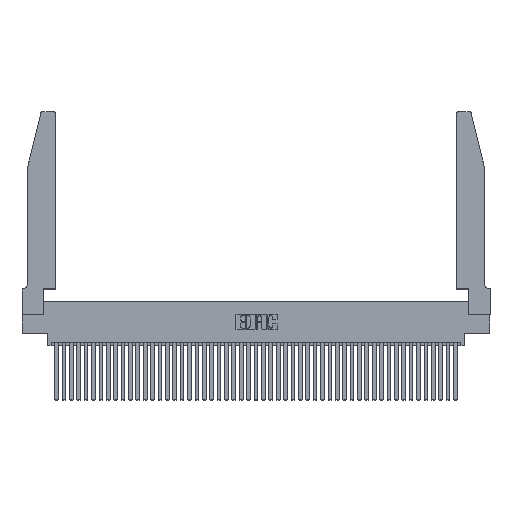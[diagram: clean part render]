
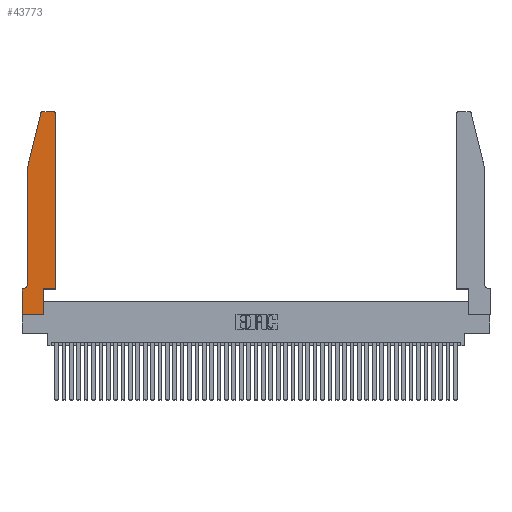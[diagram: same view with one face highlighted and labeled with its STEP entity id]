
A CAD part, top view. The second image highlights one B-rep face of the part: STEP entity #43773.
In plain terms, the highlighted planar face has unit normal (0, 0, 1).
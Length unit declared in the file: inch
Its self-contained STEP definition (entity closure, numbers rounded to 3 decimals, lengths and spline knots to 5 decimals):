
#273 = CARTESIAN_POINT ( 'NONE',  ( 0.4205, 2.75, 0.37 ) ) ;
#362 = DIRECTION ( 'NONE',  ( 0., -1., 0. ) ) ;
#999 = PLANE ( 'NONE',  #20198 ) ;
#1131 = DIRECTION ( 'NONE',  ( 0., 1., 0. ) ) ;
#1337 = DIRECTION ( 'NONE',  ( -1., 0., 0. ) ) ;
#2720 = LINE ( 'NONE', #8926, #39398 ) ;
#3730 = VECTOR ( 'NONE', #14422, 39.37008 ) ;
#4955 = DIRECTION ( 'NONE',  ( -1., 0., 0. ) ) ;
#5013 = ORIENTED_EDGE ( 'NONE', *, *, #34243, .T. ) ;
#5047 = EDGE_CURVE ( 'NONE', #11377, #32336, #18313, .T. ) ;
#5976 = VERTEX_POINT ( 'NONE', #34048 ) ;
#5987 = CARTESIAN_POINT ( 'NONE',  ( 0.2865, 0.35, 0.37 ) ) ;
#6213 = DIRECTION ( 'NONE',  ( 1., 0., 0. ) ) ;
#6577 = EDGE_CURVE ( 'NONE', #20558, #6894, #37673, .T. ) ;
#6894 = VERTEX_POINT ( 'NONE', #27374 ) ;
#7267 = VERTEX_POINT ( 'NONE', #13589 ) ;
#8099 = DIRECTION ( 'NONE',  ( -1., 0., 0. ) ) ;
#8887 = ORIENTED_EDGE ( 'NONE', *, *, #29175, .T. ) ;
#8895 = VERTEX_POINT ( 'NONE', #28972 ) ;
#8926 = CARTESIAN_POINT ( 'NONE',  ( 0.0755, 2., 0.37 ) ) ;
#9089 = ORIENTED_EDGE ( 'NONE', *, *, #15522, .T. ) ;
#9183 = LINE ( 'NONE', #5987, #32530 ) ;
#9384 = VECTOR ( 'NONE', #6213, 39.37008 ) ;
#9805 = ORIENTED_EDGE ( 'NONE', *, *, #21451, .T. ) ;
#9824 = CARTESIAN_POINT ( 'NONE',  ( 0.284, 2.72, 0.37 ) ) ;
#10603 = AXIS2_PLACEMENT_3D ( 'NONE', #9824, #34579, #20391 ) ;
#11182 = CIRCLE ( 'NONE', #27016, 0.03 ) ;
#11377 = VERTEX_POINT ( 'NONE', #30159 ) ;
#11873 = AXIS2_PLACEMENT_3D ( 'NONE', #33204, #11898, #1337 ) ;
#11898 = DIRECTION ( 'NONE',  ( 0., 0., -1. ) ) ;
#12646 = DIRECTION ( 'NONE',  ( 0., 1., 0. ) ) ;
#13589 = CARTESIAN_POINT ( 'NONE',  ( 0.2865, 0., 0.37 ) ) ;
#14422 = DIRECTION ( 'NONE',  ( -0.239, -0.971, 0. ) ) ;
#14531 = VECTOR ( 'NONE', #4955, 39.37008 ) ;
#15015 = CARTESIAN_POINT ( 'NONE',  ( 0., 0., 0.37 ) ) ;
#15304 = DIRECTION ( 'NONE',  ( 0., 0., 1. ) ) ;
#15387 = CIRCLE ( 'NONE', #11873, 0.07 ) ;
#15401 = VERTEX_POINT ( 'NONE', #40515 ) ;
#15522 = EDGE_CURVE ( 'NONE', #7267, #41668, #9183, .T. ) ;
#16374 = CIRCLE ( 'NONE', #10603, 0.03 ) ;
#17278 = ORIENTED_EDGE ( 'NONE', *, *, #20208, .T. ) ;
#18263 = DIRECTION ( 'NONE',  ( 1., 0., 0. ) ) ;
#18313 = LINE ( 'NONE', #43938, #21668 ) ;
#19512 = CARTESIAN_POINT ( 'NONE',  ( 0.4505, 0.35, 0.37 ) ) ;
#20067 = EDGE_LOOP ( 'NONE', ( #26742, #17278, #45727, #5013, #36263, #21174, #25155, #35264, #9089, #24093, #8887, #9805 ) ) ;
#20115 = DIRECTION ( 'NONE',  ( 0., -1., 0. ) ) ;
#20198 = AXIS2_PLACEMENT_3D ( 'NONE', #26035, #15304, #22627 ) ;
#20208 = EDGE_CURVE ( 'NONE', #8895, #20558, #16374, .T. ) ;
#20391 = DIRECTION ( 'NONE',  ( 1., 0., 0. ) ) ;
#20558 = VERTEX_POINT ( 'NONE', #22416 ) ;
#21174 = ORIENTED_EDGE ( 'NONE', *, *, #5047, .T. ) ;
#21451 = EDGE_CURVE ( 'NONE', #5976, #32755, #11182, .T. ) ;
#21668 = VECTOR ( 'NONE', #8099, 39.37008 ) ;
#22416 = CARTESIAN_POINT ( 'NONE',  ( 0.25487, 2.72718, 0.37 ) ) ;
#22627 = DIRECTION ( 'NONE',  ( 1., 0., 0. ) ) ;
#23021 = EDGE_CURVE ( 'NONE', #41668, #23641, #27775, .T. ) ;
#23641 = VERTEX_POINT ( 'NONE', #19512 ) ;
#23778 = CARTESIAN_POINT ( 'NONE',  ( 0., 0., 0.37 ) ) ;
#24093 = ORIENTED_EDGE ( 'NONE', *, *, #23021, .T. ) ;
#24389 = CARTESIAN_POINT ( 'NONE',  ( 0.0755, 2., 0.37 ) ) ;
#24399 = LINE ( 'NONE', #23778, #9384 ) ;
#24621 = FACE_OUTER_BOUND ( 'NONE', #20067, .T. ) ;
#25155 = ORIENTED_EDGE ( 'NONE', *, *, #38275, .T. ) ;
#25812 = CARTESIAN_POINT ( 'NONE',  ( 0.4205, 2.72, 0.37 ) ) ;
#25898 = CARTESIAN_POINT ( 'NONE',  ( 0.4505, 0.35, 0.37 ) ) ;
#26035 = CARTESIAN_POINT ( 'NONE',  ( 0., 0.35, 0.37 ) ) ;
#26742 = ORIENTED_EDGE ( 'NONE', *, *, #31777, .T. ) ;
#26892 = EDGE_CURVE ( 'NONE', #15401, #7267, #24399, .T. ) ;
#27016 = AXIS2_PLACEMENT_3D ( 'NONE', #25812, #34556, #32589 ) ;
#27374 = CARTESIAN_POINT ( 'NONE',  ( 0.0755, 2., 0.37 ) ) ;
#27775 = LINE ( 'NONE', #25898, #39424 ) ;
#28972 = CARTESIAN_POINT ( 'NONE',  ( 0.284, 2.75, 0.37 ) ) ;
#29175 = EDGE_CURVE ( 'NONE', #23641, #5976, #37535, .T. ) ;
#30159 = CARTESIAN_POINT ( 'NONE',  ( 0.0055, 0.35, 0.37 ) ) ;
#30520 = CARTESIAN_POINT ( 'NONE',  ( 0.2865, 0.35, 0.37 ) ) ;
#31777 = EDGE_CURVE ( 'NONE', #32755, #8895, #37366, .T. ) ;
#32336 = VERTEX_POINT ( 'NONE', #40829 ) ;
#32478 = VERTEX_POINT ( 'NONE', #34439 ) ;
#32530 = VECTOR ( 'NONE', #12646, 39.37008 ) ;
#32589 = DIRECTION ( 'NONE',  ( 1., 0., 0. ) ) ;
#32755 = VERTEX_POINT ( 'NONE', #273 ) ;
#33204 = CARTESIAN_POINT ( 'NONE',  ( 0.0055, 0.42, 0.37 ) ) ;
#34048 = CARTESIAN_POINT ( 'NONE',  ( 0.4505, 2.72, 0.37 ) ) ;
#34243 = EDGE_CURVE ( 'NONE', #6894, #32478, #2720, .T. ) ;
#34439 = CARTESIAN_POINT ( 'NONE',  ( 0.0755, 0.42, 0.37 ) ) ;
#34556 = DIRECTION ( 'NONE',  ( 0., 0., 1. ) ) ;
#34579 = DIRECTION ( 'NONE',  ( 0., 0., 1. ) ) ;
#35264 = ORIENTED_EDGE ( 'NONE', *, *, #26892, .T. ) ;
#36263 = ORIENTED_EDGE ( 'NONE', *, *, #45438, .T. ) ;
#36679 = CARTESIAN_POINT ( 'NONE',  ( 0.2605, 2.75, 0.37 ) ) ;
#37366 = LINE ( 'NONE', #36679, #14531 ) ;
#37535 = LINE ( 'NONE', #44102, #38084 ) ;
#37673 = LINE ( 'NONE', #24389, #3730 ) ;
#38084 = VECTOR ( 'NONE', #1131, 39.37008 ) ;
#38275 = EDGE_CURVE ( 'NONE', #32336, #15401, #41816, .T. ) ;
#39398 = VECTOR ( 'NONE', #20115, 39.37008 ) ;
#39424 = VECTOR ( 'NONE', #18263, 39.37008 ) ;
#40515 = CARTESIAN_POINT ( 'NONE',  ( 0., 0., 0.37 ) ) ;
#40829 = CARTESIAN_POINT ( 'NONE',  ( 0., 0.35, 0.37 ) ) ;
#41668 = VERTEX_POINT ( 'NONE', #30520 ) ;
#41816 = LINE ( 'NONE', #15015, #44592 ) ;
#43773 = ADVANCED_FACE ( 'NONE', ( #24621 ), #999, .T. ) ;
#43938 = CARTESIAN_POINT ( 'NONE',  ( 0.0755, 0.35, 0.37 ) ) ;
#44102 = CARTESIAN_POINT ( 'NONE',  ( 0.4505, 0.35, 0.37 ) ) ;
#44592 = VECTOR ( 'NONE', #362, 39.37008 ) ;
#45438 = EDGE_CURVE ( 'NONE', #32478, #11377, #15387, .T. ) ;
#45727 = ORIENTED_EDGE ( 'NONE', *, *, #6577, .T. ) ;
